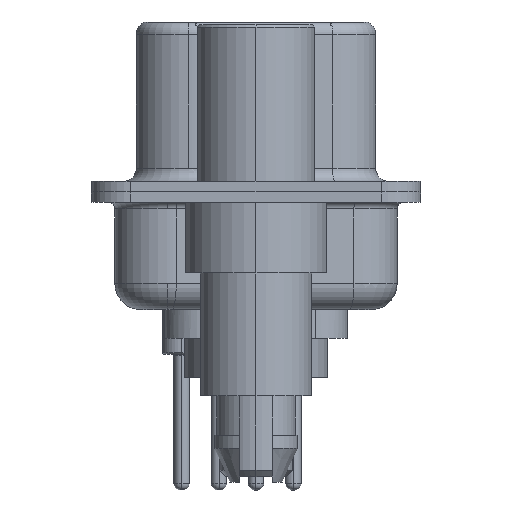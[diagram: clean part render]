
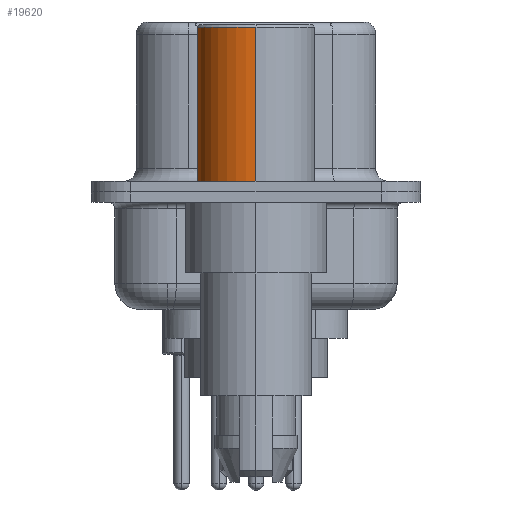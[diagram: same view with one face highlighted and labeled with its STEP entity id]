
A CAD part, left-side view. The second image highlights one B-rep face of the part: STEP entity #19620.
In plain terms, the highlighted cylindrical face has radius 2.25 mm (diameter 4.5 mm), a partial arc.
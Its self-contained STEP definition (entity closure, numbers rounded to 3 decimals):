
#8 = VECTOR ( 'NONE', #452, 1000. ) ;
#89 = DIRECTION ( 'NONE',  ( 1., 0., 0. ) ) ;
#100 = EDGE_CURVE ( 'NONE', #12719, #5271, #1451, .T. ) ;
#177 = CIRCLE ( 'NONE', #6550, 2.25 ) ;
#386 = DIRECTION ( 'NONE',  ( 1., 0., 0. ) ) ;
#452 = DIRECTION ( 'NONE',  ( 0., 0., 1. ) ) ;
#1003 = CARTESIAN_POINT ( 'NONE',  ( 0., 0., 0.4 ) ) ;
#1451 = LINE ( 'NONE', #15854, #5667 ) ;
#1456 = ORIENTED_EDGE ( 'NONE', *, *, #17631, .T. ) ;
#2551 = DIRECTION ( 'NONE',  ( 1., 0., 0. ) ) ;
#4161 = ORIENTED_EDGE ( 'NONE', *, *, #10688, .F. ) ;
#4800 = CYLINDRICAL_SURFACE ( 'NONE', #6577, 2.25 ) ;
#5190 = ORIENTED_EDGE ( 'NONE', *, *, #8970, .F. ) ;
#5271 = VERTEX_POINT ( 'NONE', #14398 ) ;
#5667 = VECTOR ( 'NONE', #20418, 1000. ) ;
#6550 = AXIS2_PLACEMENT_3D ( 'NONE', #1003, #12090, #2551 ) ;
#6577 = AXIS2_PLACEMENT_3D ( 'NONE', #11142, #12788, #89 ) ;
#6757 = CARTESIAN_POINT ( 'NONE',  ( -2.25, 0., 0.4 ) ) ;
#8970 = EDGE_CURVE ( 'NONE', #17852, #5271, #11156, .T. ) ;
#9517 = FACE_OUTER_BOUND ( 'NONE', #18509, .T. ) ;
#9862 = DIRECTION ( 'NONE',  ( 0., 0., 1. ) ) ;
#9927 = CARTESIAN_POINT ( 'NONE',  ( 2.25, 0., 0.581 ) ) ;
#10688 = EDGE_CURVE ( 'NONE', #18478, #17852, #11125, .T. ) ;
#11125 = LINE ( 'NONE', #9927, #8 ) ;
#11140 = CARTESIAN_POINT ( 'NONE',  ( 2.25, 0., 6.3 ) ) ;
#11142 = CARTESIAN_POINT ( 'NONE',  ( 0., 0., 0.581 ) ) ;
#11156 = CIRCLE ( 'NONE', #15420, 2.25 ) ;
#12090 = DIRECTION ( 'NONE',  ( 0., 0., 1. ) ) ;
#12719 = VERTEX_POINT ( 'NONE', #6757 ) ;
#12788 = DIRECTION ( 'NONE',  ( 0., 0., 1. ) ) ;
#14398 = CARTESIAN_POINT ( 'NONE',  ( -2.25, 0., 6.3 ) ) ;
#15420 = AXIS2_PLACEMENT_3D ( 'NONE', #19569, #9862, #386 ) ;
#15854 = CARTESIAN_POINT ( 'NONE',  ( -2.25, 0., 0.581 ) ) ;
#15931 = ORIENTED_EDGE ( 'NONE', *, *, #100, .T. ) ;
#17631 = EDGE_CURVE ( 'NONE', #18478, #12719, #177, .T. ) ;
#17825 = CARTESIAN_POINT ( 'NONE',  ( 2.25, 0., 0.4 ) ) ;
#17852 = VERTEX_POINT ( 'NONE', #11140 ) ;
#18478 = VERTEX_POINT ( 'NONE', #17825 ) ;
#18509 = EDGE_LOOP ( 'NONE', ( #1456, #15931, #5190, #4161 ) ) ;
#19569 = CARTESIAN_POINT ( 'NONE',  ( 0., 0., 6.3 ) ) ;
#19620 = ADVANCED_FACE ( 'NONE', ( #9517 ), #4800, .T. ) ;
#20418 = DIRECTION ( 'NONE',  ( 0., 0., 1. ) ) ;
